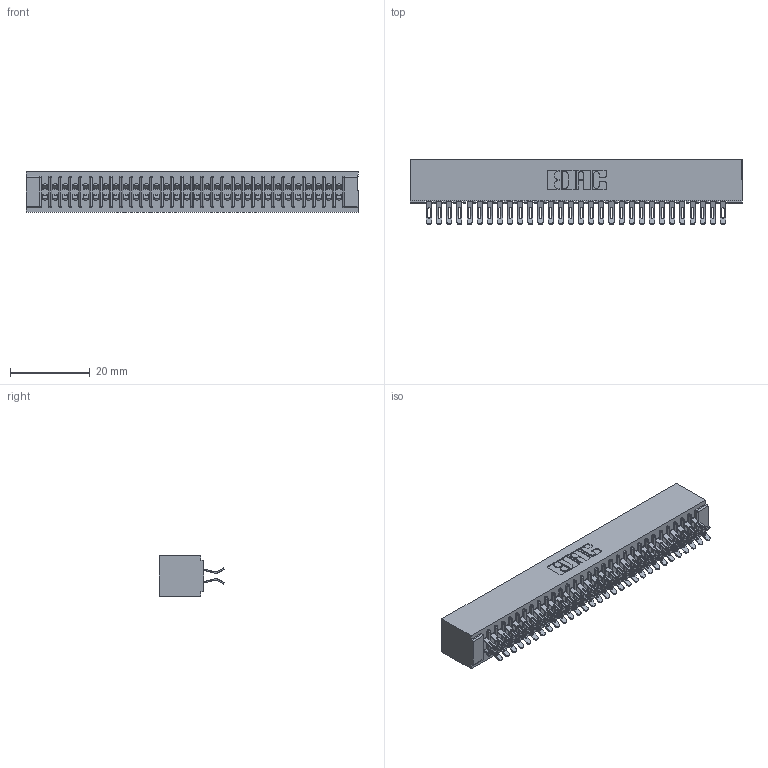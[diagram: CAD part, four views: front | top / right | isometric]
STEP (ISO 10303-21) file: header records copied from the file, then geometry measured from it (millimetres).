
FILE_DESCRIPTION (( 'STEP AP203' ), '1' );
FILE_NAME ('391-060-555-201.STEP', '2018-08-09T12:43:20', ( '' ), ( '' ), 'SwSTEP 2.0', 'SolidWorks 2016', '' );
FILE_SCHEMA (( 'CONFIG_CONTROL_DESIGN' ));
Length unit declared in the file: inch
Products named in the file (3): 341 Part_No Mounting Lugs; 341-292-001_341-292-155; 391-060-555-201
Assembly tree (61 placements, depth 2):
  391-060-555-201
    341 Part_No Mounting Lugs
    341-292-001_341-292-155  x60
Bounding box: 83.19 x 16.31 x 10.16 mm (x, y, z)
Volume: 6444.3 mm3; surface area: 12212.6 mm2
Topology: 61 solids, 61 shells, 4788 faces, 14302 edges, 9310 vertices
Faces by surface type: plane 2584, cylinder 2084, sphere 62, torus 58
Entity records: 38097 total; most frequent: CARTESIAN_POINT 6348, ORIENTED_EDGE 6296, DIRECTION 6158, EDGE_CURVE 3148, VECTOR 2518, LINE 2518, VERTEX_POINT 1994, AXIS2_PLACEMENT_3D 1820
